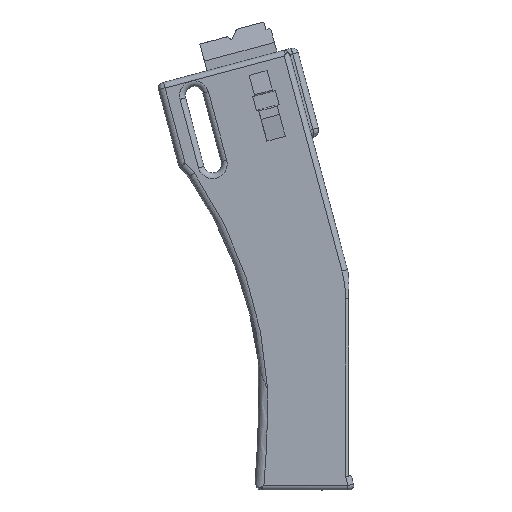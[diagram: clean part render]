
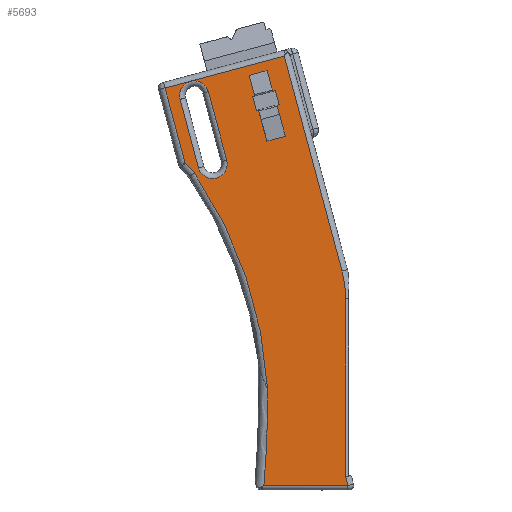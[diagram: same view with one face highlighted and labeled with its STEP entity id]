
A CAD part, front view. The second image highlights one B-rep face of the part: STEP entity #5693.
In plain terms, the highlighted planar face has unit normal (0, -1, 0).
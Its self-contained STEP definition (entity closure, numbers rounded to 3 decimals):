
#151=FACE_BOUND('',#1145,.T.);
#152=FACE_BOUND('',#1146,.T.);
#627=CIRCLE('',#6097,188.433);
#628=CIRCLE('',#6098,482.501);
#629=CIRCLE('',#6099,47.5);
#630=CIRCLE('',#6100,6.5);
#631=CIRCLE('',#6101,6.5);
#797=FACE_OUTER_BOUND('',#1144,.T.);
#1144=EDGE_LOOP('',(#4010,#4011,#4012,#4013,#4014,#4015,#4016,#4017,#4018,
#4019));
#1145=EDGE_LOOP('',(#4020,#4021,#4022,#4023,#4024,#4025,#4026,#4027,#4028,
#4029,#4030,#4031));
#1146=EDGE_LOOP('',(#4032,#4033,#4034,#4035));
#1483=LINE('',#7969,#1872);
#1493=LINE('',#8132,#1882);
#1500=LINE('',#8151,#1889);
#1503=LINE('',#8156,#1892);
#1515=LINE('',#8278,#1904);
#1546=LINE('',#8568,#1935);
#1547=LINE('',#8570,#1936);
#1548=LINE('',#8572,#1937);
#1549=LINE('',#8577,#1938);
#1550=LINE('',#8579,#1939);
#1551=LINE('',#8582,#1940);
#1552=LINE('',#8584,#1941);
#1553=LINE('',#8586,#1942);
#1554=LINE('',#8587,#1943);
#1555=LINE('',#8589,#1944);
#1556=LINE('',#8591,#1945);
#1557=LINE('',#8593,#1946);
#1558=LINE('',#8595,#1947);
#1559=LINE('',#8596,#1948);
#1560=LINE('',#8599,#1949);
#1561=LINE('',#8603,#1950);
#1872=VECTOR('',#6576,10.);
#1882=VECTOR('',#6612,10.);
#1889=VECTOR('',#6629,10.);
#1892=VECTOR('',#6634,10.);
#1904=VECTOR('',#6672,10.);
#1935=VECTOR('',#6727,10.);
#1936=VECTOR('',#6728,10.);
#1937=VECTOR('',#6729,10.);
#1938=VECTOR('',#6734,10.);
#1939=VECTOR('',#6735,10.);
#1940=VECTOR('',#6738,10.);
#1941=VECTOR('',#6739,10.);
#1942=VECTOR('',#6740,10.);
#1943=VECTOR('',#6741,10.);
#1944=VECTOR('',#6742,10.);
#1945=VECTOR('',#6743,10.);
#1946=VECTOR('',#6744,10.);
#1947=VECTOR('',#6745,10.);
#1948=VECTOR('',#6746,10.);
#1949=VECTOR('',#6747,10.);
#1950=VECTOR('',#6750,10.);
#2292=VERTEX_POINT('',#7966);
#2293=VERTEX_POINT('',#7968);
#2311=VERTEX_POINT('',#8129);
#2312=VERTEX_POINT('',#8131);
#2318=VERTEX_POINT('',#8148);
#2319=VERTEX_POINT('',#8150);
#2320=VERTEX_POINT('',#8154);
#2335=VERTEX_POINT('',#8275);
#2336=VERTEX_POINT('',#8277);
#2403=VERTEX_POINT('',#8567);
#2404=VERTEX_POINT('',#8569);
#2405=VERTEX_POINT('',#8571);
#2406=VERTEX_POINT('',#8573);
#2407=VERTEX_POINT('',#8575);
#2408=VERTEX_POINT('',#8578);
#2409=VERTEX_POINT('',#8581);
#2410=VERTEX_POINT('',#8583);
#2411=VERTEX_POINT('',#8585);
#2412=VERTEX_POINT('',#8588);
#2413=VERTEX_POINT('',#8590);
#2414=VERTEX_POINT('',#8592);
#2415=VERTEX_POINT('',#8594);
#2416=VERTEX_POINT('',#8597);
#2417=VERTEX_POINT('',#8598);
#2418=VERTEX_POINT('',#8600);
#2419=VERTEX_POINT('',#8602);
#2887=EDGE_CURVE('',#2292,#2293,#1483,.T.);
#2910=EDGE_CURVE('',#2312,#2311,#1493,.T.);
#2919=EDGE_CURVE('',#2319,#2318,#1500,.T.);
#2922=EDGE_CURVE('',#2320,#2318,#1503,.T.);
#2945=EDGE_CURVE('',#2335,#2336,#1515,.T.);
#3019=EDGE_CURVE('',#2335,#2403,#1546,.T.);
#3020=EDGE_CURVE('',#2404,#2403,#1547,.T.);
#3021=EDGE_CURVE('',#2405,#2404,#1548,.T.);
#3022=EDGE_CURVE('',#2406,#2405,#627,.T.);
#3023=EDGE_CURVE('',#2407,#2406,#628,.T.);
#3024=EDGE_CURVE('',#2293,#2407,#1549,.T.);
#3025=EDGE_CURVE('',#2408,#2292,#1550,.T.);
#3026=EDGE_CURVE('',#2336,#2408,#629,.T.);
#3027=EDGE_CURVE('',#2320,#2409,#1551,.T.);
#3028=EDGE_CURVE('',#2409,#2410,#1552,.T.);
#3029=EDGE_CURVE('',#2410,#2411,#1553,.T.);
#3030=EDGE_CURVE('',#2312,#2411,#1554,.T.);
#3031=EDGE_CURVE('',#2311,#2412,#1555,.T.);
#3032=EDGE_CURVE('',#2412,#2413,#1556,.T.);
#3033=EDGE_CURVE('',#2414,#2413,#1557,.T.);
#3034=EDGE_CURVE('',#2414,#2415,#1558,.T.);
#3035=EDGE_CURVE('',#2415,#2319,#1559,.T.);
#3036=EDGE_CURVE('',#2416,#2417,#1560,.T.);
#3037=EDGE_CURVE('',#2418,#2416,#630,.T.);
#3038=EDGE_CURVE('',#2419,#2418,#1561,.T.);
#3039=EDGE_CURVE('',#2417,#2419,#631,.T.);
#4010=ORIENTED_EDGE('',*,*,#3019,.T.);
#4011=ORIENTED_EDGE('',*,*,#3020,.F.);
#4012=ORIENTED_EDGE('',*,*,#3021,.F.);
#4013=ORIENTED_EDGE('',*,*,#3022,.F.);
#4014=ORIENTED_EDGE('',*,*,#3023,.F.);
#4015=ORIENTED_EDGE('',*,*,#3024,.F.);
#4016=ORIENTED_EDGE('',*,*,#2887,.F.);
#4017=ORIENTED_EDGE('',*,*,#3025,.F.);
#4018=ORIENTED_EDGE('',*,*,#3026,.F.);
#4019=ORIENTED_EDGE('',*,*,#2945,.F.);
#4020=ORIENTED_EDGE('',*,*,#3027,.T.);
#4021=ORIENTED_EDGE('',*,*,#3028,.T.);
#4022=ORIENTED_EDGE('',*,*,#3029,.T.);
#4023=ORIENTED_EDGE('',*,*,#3030,.F.);
#4024=ORIENTED_EDGE('',*,*,#2910,.T.);
#4025=ORIENTED_EDGE('',*,*,#3031,.T.);
#4026=ORIENTED_EDGE('',*,*,#3032,.T.);
#4027=ORIENTED_EDGE('',*,*,#3033,.F.);
#4028=ORIENTED_EDGE('',*,*,#3034,.T.);
#4029=ORIENTED_EDGE('',*,*,#3035,.T.);
#4030=ORIENTED_EDGE('',*,*,#2919,.T.);
#4031=ORIENTED_EDGE('',*,*,#2922,.F.);
#4032=ORIENTED_EDGE('',*,*,#3036,.F.);
#4033=ORIENTED_EDGE('',*,*,#3037,.F.);
#4034=ORIENTED_EDGE('',*,*,#3038,.F.);
#4035=ORIENTED_EDGE('',*,*,#3039,.F.);
#5542=PLANE('',#6096);
#5693=ADVANCED_FACE('',(#797,#151,#152),#5542,.T.);
#6096=AXIS2_PLACEMENT_3D('',#8566,#6725,#6726);
#6097=AXIS2_PLACEMENT_3D('',#8574,#6730,#6731);
#6098=AXIS2_PLACEMENT_3D('',#8576,#6732,#6733);
#6099=AXIS2_PLACEMENT_3D('',#8580,#6736,#6737);
#6100=AXIS2_PLACEMENT_3D('',#8601,#6748,#6749);
#6101=AXIS2_PLACEMENT_3D('',#8604,#6751,#6752);
#6576=DIRECTION('',(0.,0.,-1.));
#6612=DIRECTION('',(0.,0.,-1.));
#6629=DIRECTION('',(0.,0.,1.));
#6634=DIRECTION('',(-1.,0.,0.));
#6672=DIRECTION('',(0.,0.,-1.));
#6725=DIRECTION('center_axis',(0.,-1.,0.));
#6726=DIRECTION('ref_axis',(1.,0.,0.));
#6727=DIRECTION('',(-1.,0.,0.));
#6728=DIRECTION('',(0.,0.,1.));
#6729=DIRECTION('',(-0.475,0.,0.88));
#6730=DIRECTION('center_axis',(0.,-1.,0.));
#6731=DIRECTION('ref_axis',(0.999,0.,-0.05));
#6732=DIRECTION('center_axis',(0.,-1.,0.));
#6733=DIRECTION('ref_axis',(0.966,0.,-0.259));
#6734=DIRECTION('',(-0.966,0.,0.259));
#6735=DIRECTION('',(-0.259,0.,-0.966));
#6736=DIRECTION('center_axis',(0.,1.,0.));
#6737=DIRECTION('ref_axis',(0.991,0.,-0.131));
#6738=DIRECTION('',(0.,0.,-1.));
#6739=DIRECTION('',(1.,0.,0.));
#6740=DIRECTION('',(0.,0.,-1.));
#6741=DIRECTION('',(1.,0.,0.));
#6742=DIRECTION('',(-1.,0.,0.));
#6743=DIRECTION('',(0.,0.,1.));
#6744=DIRECTION('',(1.,0.,0.));
#6745=DIRECTION('',(0.,0.,1.));
#6746=DIRECTION('',(1.,0.,0.));
#6747=DIRECTION('',(0.,0.,-1.));
#6748=DIRECTION('center_axis',(0.,-1.,0.));
#6749=DIRECTION('ref_axis',(0.,0.,
1.));
#6750=DIRECTION('',(0.,0.,1.));
#6751=DIRECTION('center_axis',(0.,-1.,0.));
#6752=DIRECTION('ref_axis',(0.,0.,-1.));
#7966=CARTESIAN_POINT('',(481.835,-39.877,-155.995));
#7968=CARTESIAN_POINT('',(481.835,-39.877,-160.139));
#7969=CARTESIAN_POINT('',(481.835,-39.877,-61.154));
#8129=CARTESIAN_POINT('',(495.059,-39.877,-3.459));
#8131=CARTESIAN_POINT('',(495.059,-39.877,10.83));
#8132=CARTESIAN_POINT('',(495.059,-39.877,-32.194));
#8148=CARTESIAN_POINT('',(486.559,-39.877,26.753));
#8150=CARTESIAN_POINT('',(486.559,-39.877,17.253));
#8151=CARTESIAN_POINT('',(486.559,-39.877,-19.463));
#8154=CARTESIAN_POINT('',(494.809,-39.877,26.753));
#8156=CARTESIAN_POINT('',(495.559,-39.877,26.753));
#8275=CARTESIAN_POINT('',(503.835,-39.877,30.987));
#8277=CARTESIAN_POINT('',(503.835,-39.877,-67.636));
#8278=CARTESIAN_POINT('',(503.835,-39.877,-20.154));
#8566=CARTESIAN_POINT('Origin',(466.451,-39.877,-60.928));
#8567=CARTESIAN_POINT('',(449.124,-39.877,30.987));
#8568=CARTESIAN_POINT('',(503.124,-39.877,30.987));
#8569=CARTESIAN_POINT('',(449.124,-39.877,-3.618));
#8570=CARTESIAN_POINT('',(449.124,-39.877,-60.891));
#8571=CARTESIAN_POINT('',(451.876,-39.877,-8.711));
#8572=CARTESIAN_POINT('',(460.138,-39.877,-23.997));
#8573=CARTESIAN_POINT('',(458.443,-39.877,-109.929));
#8574=CARTESIAN_POINT('Origin',(274.06,-39.877,-71.069));
#8575=CARTESIAN_POINT('',(445.854,-39.877,-150.498));
#8576=CARTESIAN_POINT('Origin',(-8.23,-39.877,12.642));
#8577=CARTESIAN_POINT('',(442.652,-39.877,-149.64));
#8578=CARTESIAN_POINT('',(502.217,-39.877,-79.93));
#8579=CARTESIAN_POINT('',(504.246,-39.877,-72.357));
#8580=CARTESIAN_POINT('Origin',(456.335,-39.877,-67.636));
#8581=CARTESIAN_POINT('',(494.809,-39.877,17.253));
#8582=CARTESIAN_POINT('',(494.809,-39.877,-19.463));
#8583=CARTESIAN_POINT('',(496.059,-39.877,17.253));
#8584=CARTESIAN_POINT('',(492.107,-39.877,17.253));
#8585=CARTESIAN_POINT('',(496.059,-39.877,10.83));
#8586=CARTESIAN_POINT('',(496.059,-39.877,-25.769));
#8587=CARTESIAN_POINT('',(492.107,-39.877,10.83));
#8588=CARTESIAN_POINT('',(486.642,-39.877,-3.459));
#8589=CARTESIAN_POINT('',(478.651,-39.877,-3.459));
#8590=CARTESIAN_POINT('',(486.642,-39.877,10.83));
#8591=CARTESIAN_POINT('',(486.642,-39.877,8.641));
#8592=CARTESIAN_POINT('',(485.642,-39.877,10.83));
#8593=CARTESIAN_POINT('',(492.107,-39.877,10.83));
#8594=CARTESIAN_POINT('',(485.642,-39.877,17.253));
#8595=CARTESIAN_POINT('',(485.642,-39.877,-22.932));
#8596=CARTESIAN_POINT('',(492.107,-39.877,17.253));
#8597=CARTESIAN_POINT('',(454.256,-39.877,24.426));
#8598=CARTESIAN_POINT('',(454.256,-39.877,-7.001));
#8599=CARTESIAN_POINT('',(454.256,-39.877,-33.965));
#8600=CARTESIAN_POINT('',(467.256,-39.877,24.426));
#8601=CARTESIAN_POINT('Origin',(460.756,-39.877,24.426));
#8602=CARTESIAN_POINT('',(467.256,-39.877,-7.001));
#8603=CARTESIAN_POINT('',(467.256,-39.877,-18.251));
#8604=CARTESIAN_POINT('Origin',(460.756,-39.877,-7.001));
